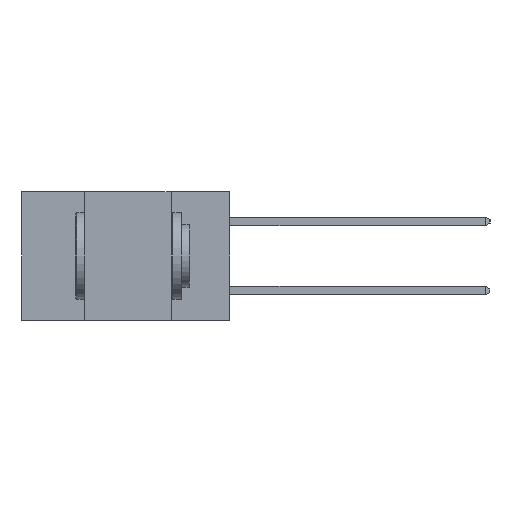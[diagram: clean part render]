
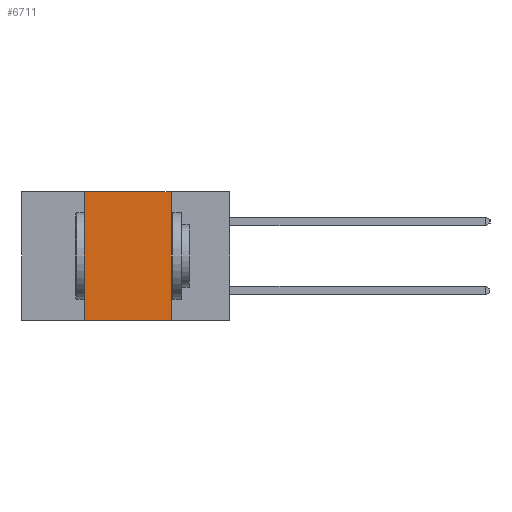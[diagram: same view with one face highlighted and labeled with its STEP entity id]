
A CAD part, left-side view. The second image highlights one B-rep face of the part: STEP entity #6711.
In plain terms, the highlighted planar face has unit normal (-1, 0, 0).
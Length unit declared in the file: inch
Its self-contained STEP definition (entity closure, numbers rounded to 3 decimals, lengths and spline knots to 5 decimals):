
#501 = EDGE_CURVE ( 'NONE', #15733, #1683, #20674, .T. ) ;
#725 = EDGE_CURVE ( 'NONE', #1683, #18614, #9733, .T. ) ;
#1267 = CARTESIAN_POINT ( 'NONE',  ( 0., 0.6, -0.37 ) ) ;
#1676 = EDGE_LOOP ( 'NONE', ( #8266, #3927, #26368, #4593 ) ) ;
#1683 = VERTEX_POINT ( 'NONE', #4979 ) ;
#2922 = DIRECTION ( 'NONE',  ( 0., -1., 0. ) ) ;
#3802 = LINE ( 'NONE', #1267, #19431 ) ;
#3803 = VERTEX_POINT ( 'NONE', #9766 ) ;
#3927 = ORIENTED_EDGE ( 'NONE', *, *, #725, .F. ) ;
#4593 = ORIENTED_EDGE ( 'NONE', *, *, #5695, .T. ) ;
#4979 = CARTESIAN_POINT ( 'NONE',  ( 0., 0.42, 0. ) ) ;
#5211 = CARTESIAN_POINT ( 'NONE',  ( 0., 0.17, 0. ) ) ;
#5509 = VECTOR ( 'NONE', #13745, 39.37008 ) ;
#5695 = EDGE_CURVE ( 'NONE', #15733, #3803, #3802, .T. ) ;
#6711 = ADVANCED_FACE ( 'NONE', ( #16747 ), #14800, .F. ) ;
#7554 = AXIS2_PLACEMENT_3D ( 'NONE', #15975, #14698, #14684 ) ;
#8266 = ORIENTED_EDGE ( 'NONE', *, *, #10519, .F. ) ;
#8278 = CARTESIAN_POINT ( 'NONE',  ( 0., 0.42, -0.37 ) ) ;
#8765 = CARTESIAN_POINT ( 'NONE',  ( 0., 0.17, 0. ) ) ;
#9733 = LINE ( 'NONE', #14649, #20327 ) ;
#9766 = CARTESIAN_POINT ( 'NONE',  ( 0., 0.17, -0.37 ) ) ;
#10519 = EDGE_CURVE ( 'NONE', #18614, #3803, #16201, .T. ) ;
#13745 = DIRECTION ( 'NONE',  ( 0., 0., -1. ) ) ;
#14649 = CARTESIAN_POINT ( 'NONE',  ( 0., 0.6, 0. ) ) ;
#14684 = DIRECTION ( 'NONE',  ( 0., 0., -1. ) ) ;
#14698 = DIRECTION ( 'NONE',  ( 1., 0., 0. ) ) ;
#14800 = PLANE ( 'NONE',  #7554 ) ;
#15096 = VECTOR ( 'NONE', #24757, 39.37008 ) ;
#15733 = VERTEX_POINT ( 'NONE', #8278 ) ;
#15975 = CARTESIAN_POINT ( 'NONE',  ( 0., 0.6, 0. ) ) ;
#16201 = LINE ( 'NONE', #5211, #5509 ) ;
#16624 = DIRECTION ( 'NONE',  ( 0., -1., 0. ) ) ;
#16747 = FACE_OUTER_BOUND ( 'NONE', #1676, .T. ) ;
#18614 = VERTEX_POINT ( 'NONE', #8765 ) ;
#19431 = VECTOR ( 'NONE', #2922, 39.37008 ) ;
#20327 = VECTOR ( 'NONE', #16624, 39.37008 ) ;
#20674 = LINE ( 'NONE', #24248, #15096 ) ;
#24248 = CARTESIAN_POINT ( 'NONE',  ( 0., 0.42, 0. ) ) ;
#24757 = DIRECTION ( 'NONE',  ( 0., 0., 1. ) ) ;
#26368 = ORIENTED_EDGE ( 'NONE', *, *, #501, .F. ) ;
